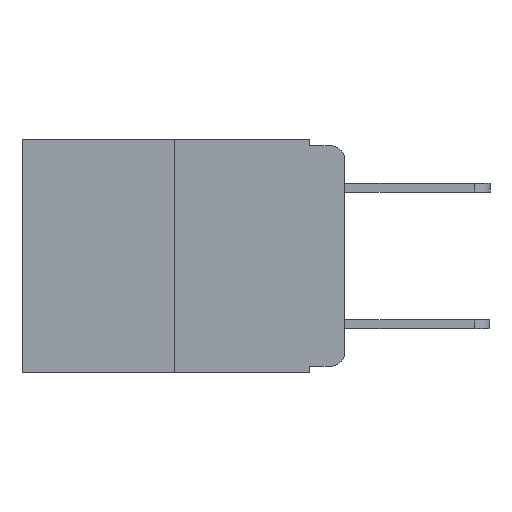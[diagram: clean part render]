
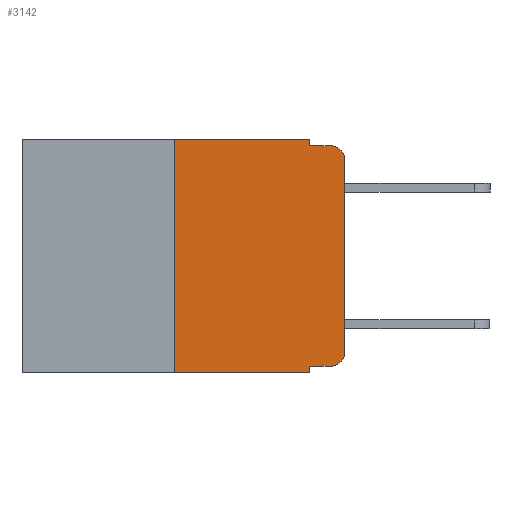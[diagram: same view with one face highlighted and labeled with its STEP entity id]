
A CAD part, left-side view. The second image highlights one B-rep face of the part: STEP entity #3142.
In plain terms, the highlighted planar face has unit normal (-1, 0, 0).
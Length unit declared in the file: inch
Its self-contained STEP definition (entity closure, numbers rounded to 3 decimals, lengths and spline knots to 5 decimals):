
#213 = DIRECTION ( 'NONE',  ( 0., 0., 1. ) ) ;
#334 = VERTEX_POINT ( 'NONE', #4701 ) ;
#577 = CARTESIAN_POINT ( 'NONE',  ( 0., 0.02, -0.333 ) ) ;
#589 = DIRECTION ( 'NONE',  ( 0., -1., 0. ) ) ;
#608 = VERTEX_POINT ( 'NONE', #4225 ) ;
#626 = DIRECTION ( 'NONE',  ( -1., 0., 0. ) ) ;
#1029 = DIRECTION ( 'NONE',  ( 0., 0., 1. ) ) ;
#1046 = VECTOR ( 'NONE', #6004, 39.37008 ) ;
#1292 = EDGE_CURVE ( 'NONE', #3904, #8742, #6204, .T. ) ;
#1376 = ORIENTED_EDGE ( 'NONE', *, *, #5428, .T. ) ;
#1404 = EDGE_CURVE ( 'NONE', #8345, #1712, #4824, .T. ) ;
#1494 = CARTESIAN_POINT ( 'NONE',  ( 0., 0.051, -0.01 ) ) ;
#1712 = VERTEX_POINT ( 'NONE', #4388 ) ;
#2265 = VECTOR ( 'NONE', #5062, 39.37008 ) ;
#2324 = FACE_OUTER_BOUND ( 'NONE', #7926, .T. ) ;
#2479 = ORIENTED_EDGE ( 'NONE', *, *, #1292, .F. ) ;
#2687 = ORIENTED_EDGE ( 'NONE', *, *, #5513, .T. ) ;
#2775 = ORIENTED_EDGE ( 'NONE', *, *, #5507, .F. ) ;
#2788 = CARTESIAN_POINT ( 'NONE',  ( 0., 0.473, 0. ) ) ;
#2994 = CIRCLE ( 'NONE', #8294, 0.02 ) ;
#3101 = CARTESIAN_POINT ( 'NONE',  ( 0., 0.051, -0.333 ) ) ;
#3142 = ADVANCED_FACE ( 'NONE', ( #2324 ), #8580, .F. ) ;
#3173 = CARTESIAN_POINT ( 'NONE',  ( 0., 0.051, -0.01 ) ) ;
#3302 = VERTEX_POINT ( 'NONE', #9542 ) ;
#3409 = DIRECTION ( 'NONE',  ( 0., 0., -1. ) ) ;
#3553 = CARTESIAN_POINT ( 'NONE',  ( 0., 0.02, -0.01 ) ) ;
#3860 = DIRECTION ( 'NONE',  ( -1., 0., 0. ) ) ;
#3904 = VERTEX_POINT ( 'NONE', #3173 ) ;
#3974 = CIRCLE ( 'NONE', #5216, 0.02 ) ;
#4225 = CARTESIAN_POINT ( 'NONE',  ( 0., 0.25, -0.343 ) ) ;
#4388 = CARTESIAN_POINT ( 'NONE',  ( 0., 0., -0.03 ) ) ;
#4571 = CARTESIAN_POINT ( 'NONE',  ( 0., 0.051, 0. ) ) ;
#4701 = CARTESIAN_POINT ( 'NONE',  ( 0., 0.051, -0.343 ) ) ;
#4719 = LINE ( 'NONE', #10693, #2265 ) ;
#4824 = LINE ( 'NONE', #10688, #8973 ) ;
#5062 = DIRECTION ( 'NONE',  ( 0., -1., 0. ) ) ;
#5114 = DIRECTION ( 'NONE',  ( 1., 0., 0. ) ) ;
#5164 = EDGE_CURVE ( 'NONE', #3302, #3904, #6243, .T. ) ;
#5191 = ORIENTED_EDGE ( 'NONE', *, *, #5233, .F. ) ;
#5216 = AXIS2_PLACEMENT_3D ( 'NONE', #8912, #3860, #9677 ) ;
#5233 = EDGE_CURVE ( 'NONE', #608, #5871, #6641, .T. ) ;
#5428 = EDGE_CURVE ( 'NONE', #9108, #7815, #4719, .T. ) ;
#5507 = EDGE_CURVE ( 'NONE', #5871, #3302, #8166, .T. ) ;
#5513 = EDGE_CURVE ( 'NONE', #7815, #8345, #2994, .T. ) ;
#5704 = VECTOR ( 'NONE', #10266, 39.37008 ) ;
#5798 = CARTESIAN_POINT ( 'NONE',  ( 0., 0., -0.313 ) ) ;
#5845 = VECTOR ( 'NONE', #589, 39.37008 ) ;
#5871 = VERTEX_POINT ( 'NONE', #10549 ) ;
#6004 = DIRECTION ( 'NONE',  ( 0., 0., -1. ) ) ;
#6144 = CARTESIAN_POINT ( 'NONE',  ( 0., 0.02, -0.313 ) ) ;
#6204 = LINE ( 'NONE', #1494, #8371 ) ;
#6218 = AXIS2_PLACEMENT_3D ( 'NONE', #2788, #5114, #3409 ) ;
#6243 = LINE ( 'NONE', #4571, #5704 ) ;
#6464 = ORIENTED_EDGE ( 'NONE', *, *, #10392, .T. ) ;
#6641 = LINE ( 'NONE', #8139, #8767 ) ;
#6957 = ORIENTED_EDGE ( 'NONE', *, *, #1404, .T. ) ;
#6975 = DIRECTION ( 'NONE',  ( 0., -1., 0. ) ) ;
#7007 = DIRECTION ( 'NONE',  ( 0., 0., -1. ) ) ;
#7329 = EDGE_CURVE ( 'NONE', #1712, #8742, #3974, .T. ) ;
#7676 = EDGE_CURVE ( 'NONE', #9108, #334, #8133, .T. ) ;
#7815 = VERTEX_POINT ( 'NONE', #577 ) ;
#7926 = EDGE_LOOP ( 'NONE', ( #6957, #9058, #2479, #9293, #2775, #5191, #6464, #7973, #1376, #2687 ) ) ;
#7973 = ORIENTED_EDGE ( 'NONE', *, *, #7676, .F. ) ;
#8133 = LINE ( 'NONE', #9975, #1046 ) ;
#8139 = CARTESIAN_POINT ( 'NONE',  ( 0., 0.25, 0. ) ) ;
#8166 = LINE ( 'NONE', #10061, #9719 ) ;
#8294 = AXIS2_PLACEMENT_3D ( 'NONE', #6144, #626, #7007 ) ;
#8345 = VERTEX_POINT ( 'NONE', #5798 ) ;
#8371 = VECTOR ( 'NONE', #10855, 39.37008 ) ;
#8580 = PLANE ( 'NONE',  #6218 ) ;
#8742 = VERTEX_POINT ( 'NONE', #3553 ) ;
#8767 = VECTOR ( 'NONE', #1029, 39.37008 ) ;
#8912 = CARTESIAN_POINT ( 'NONE',  ( 0., 0.02, -0.03 ) ) ;
#8973 = VECTOR ( 'NONE', #213, 39.37008 ) ;
#9058 = ORIENTED_EDGE ( 'NONE', *, *, #7329, .T. ) ;
#9108 = VERTEX_POINT ( 'NONE', #3101 ) ;
#9293 = ORIENTED_EDGE ( 'NONE', *, *, #5164, .F. ) ;
#9341 = CARTESIAN_POINT ( 'NONE',  ( 0., 0.473, -0.343 ) ) ;
#9542 = CARTESIAN_POINT ( 'NONE',  ( 0., 0.051, 0. ) ) ;
#9677 = DIRECTION ( 'NONE',  ( 0., 0., -1. ) ) ;
#9719 = VECTOR ( 'NONE', #6975, 39.37008 ) ;
#9975 = CARTESIAN_POINT ( 'NONE',  ( 0., 0.051, 0. ) ) ;
#10061 = CARTESIAN_POINT ( 'NONE',  ( 0., 0.473, 0. ) ) ;
#10266 = DIRECTION ( 'NONE',  ( 0., 0., -1. ) ) ;
#10319 = LINE ( 'NONE', #9341, #5845 ) ;
#10392 = EDGE_CURVE ( 'NONE', #608, #334, #10319, .T. ) ;
#10549 = CARTESIAN_POINT ( 'NONE',  ( 0., 0.25, 0. ) ) ;
#10688 = CARTESIAN_POINT ( 'NONE',  ( 0., 0., 0. ) ) ;
#10693 = CARTESIAN_POINT ( 'NONE',  ( 0., 0.051, -0.333 ) ) ;
#10855 = DIRECTION ( 'NONE',  ( 0., -1., 0. ) ) ;
